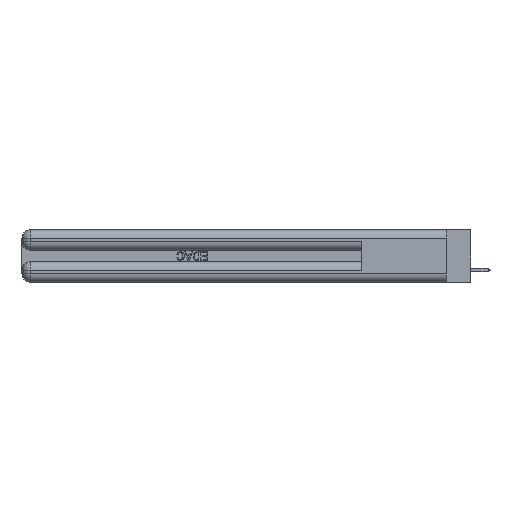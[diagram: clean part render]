
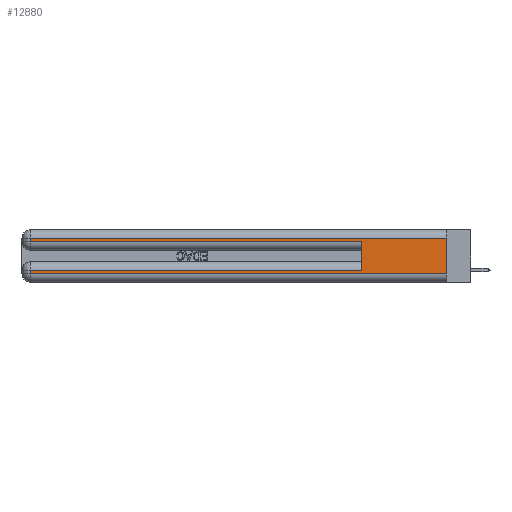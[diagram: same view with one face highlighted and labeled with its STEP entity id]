
A CAD part, left-side view. The second image highlights one B-rep face of the part: STEP entity #12880.
In plain terms, the highlighted planar face has unit normal (-1, 0, 0).
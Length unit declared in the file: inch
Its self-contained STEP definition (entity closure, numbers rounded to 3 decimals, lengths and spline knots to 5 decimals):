
#686 = EDGE_LOOP ( 'NONE', ( #40290, #36398, #44369, #18513, #11837, #49106, #40680, #31787 ) ) ;
#729 = CARTESIAN_POINT ( 'NONE',  ( 0., 0., 0.37 ) ) ;
#1629 = DIRECTION ( 'NONE',  ( 1., 0., 0. ) ) ;
#2699 = DIRECTION ( 'NONE',  ( 0., -1., 0. ) ) ;
#3109 = VECTOR ( 'NONE', #3768, 39.37008 ) ;
#3409 = VECTOR ( 'NONE', #29097, 39.37008 ) ;
#3768 = DIRECTION ( 'NONE',  ( 0., 1., 0. ) ) ;
#4962 = DIRECTION ( 'NONE',  ( 0., 0., -1. ) ) ;
#5682 = VECTOR ( 'NONE', #28118, 39.37008 ) ;
#6761 = CARTESIAN_POINT ( 'NONE',  ( 0., 2.94, 0.37 ) ) ;
#6927 = LINE ( 'NONE', #31797, #5682 ) ;
#8774 = VERTEX_POINT ( 'NONE', #41398 ) ;
#8833 = VECTOR ( 'NONE', #4962, 39.37008 ) ;
#9168 = PLANE ( 'NONE',  #35227 ) ;
#9679 = VERTEX_POINT ( 'NONE', #45547 ) ;
#10828 = VECTOR ( 'NONE', #41922, 39.37008 ) ;
#11837 = ORIENTED_EDGE ( 'NONE', *, *, #23408, .F. ) ;
#11950 = CARTESIAN_POINT ( 'NONE',  ( 0., 0., 0.31 ) ) ;
#11981 = CARTESIAN_POINT ( 'NONE',  ( 0., 2.94, 0.06 ) ) ;
#12513 = CARTESIAN_POINT ( 'NONE',  ( 0., 0., 0.085 ) ) ;
#12880 = ADVANCED_FACE ( 'NONE', ( #46481 ), #9168, .F. ) ;
#13330 = VECTOR ( 'NONE', #2699, 39.37008 ) ;
#13596 = DIRECTION ( 'NONE',  ( 0., 0., -1. ) ) ;
#17087 = VERTEX_POINT ( 'NONE', #45093 ) ;
#17309 = CARTESIAN_POINT ( 'NONE',  ( 0., 2.94, 0.085 ) ) ;
#18139 = VERTEX_POINT ( 'NONE', #26440 ) ;
#18380 = LINE ( 'NONE', #6761, #31549 ) ;
#18513 = ORIENTED_EDGE ( 'NONE', *, *, #37008, .T. ) ;
#20702 = VERTEX_POINT ( 'NONE', #29955 ) ;
#20834 = CARTESIAN_POINT ( 'NONE',  ( 0., 0., 0.37 ) ) ;
#22202 = CARTESIAN_POINT ( 'NONE',  ( 0., 2.94, 0.31 ) ) ;
#23085 = DIRECTION ( 'NONE',  ( 0., 0., -1. ) ) ;
#23408 = EDGE_CURVE ( 'NONE', #18139, #8774, #39135, .T. ) ;
#23562 = LINE ( 'NONE', #48518, #13330 ) ;
#23780 = DIRECTION ( 'NONE',  ( 0., -1., 0. ) ) ;
#23832 = LINE ( 'NONE', #12513, #3409 ) ;
#24650 = LINE ( 'NONE', #39279, #39713 ) ;
#25997 = EDGE_CURVE ( 'NONE', #27958, #32649, #18380, .T. ) ;
#26440 = CARTESIAN_POINT ( 'NONE',  ( 0., 0.6, 0.085 ) ) ;
#26708 = EDGE_CURVE ( 'NONE', #18139, #27958, #23832, .T. ) ;
#27144 = EDGE_CURVE ( 'NONE', #44528, #20702, #6927, .T. ) ;
#27958 = VERTEX_POINT ( 'NONE', #17309 ) ;
#28118 = DIRECTION ( 'NONE',  ( 0., 0., -1. ) ) ;
#29097 = DIRECTION ( 'NONE',  ( 0., 1., 0. ) ) ;
#29428 = LINE ( 'NONE', #729, #8833 ) ;
#29955 = CARTESIAN_POINT ( 'NONE',  ( 0., 2.94, 0.285 ) ) ;
#30096 = EDGE_CURVE ( 'NONE', #32649, #9679, #24650, .T. ) ;
#31350 = LINE ( 'NONE', #11950, #3109 ) ;
#31549 = VECTOR ( 'NONE', #23085, 39.37008 ) ;
#31787 = ORIENTED_EDGE ( 'NONE', *, *, #30096, .T. ) ;
#31797 = CARTESIAN_POINT ( 'NONE',  ( 0., 2.94, 0.37 ) ) ;
#32649 = VERTEX_POINT ( 'NONE', #11981 ) ;
#34162 = CARTESIAN_POINT ( 'NONE',  ( 0., 0.6, 0.145 ) ) ;
#35227 = AXIS2_PLACEMENT_3D ( 'NONE', #20834, #1629, #13596 ) ;
#36398 = ORIENTED_EDGE ( 'NONE', *, *, #42828, .T. ) ;
#37008 = EDGE_CURVE ( 'NONE', #20702, #8774, #23562, .T. ) ;
#39135 = LINE ( 'NONE', #34162, #10828 ) ;
#39279 = CARTESIAN_POINT ( 'NONE',  ( 0., 0., 0.06 ) ) ;
#39713 = VECTOR ( 'NONE', #23780, 39.37008 ) ;
#40290 = ORIENTED_EDGE ( 'NONE', *, *, #45122, .F. ) ;
#40680 = ORIENTED_EDGE ( 'NONE', *, *, #25997, .T. ) ;
#41398 = CARTESIAN_POINT ( 'NONE',  ( 0., 0.6, 0.285 ) ) ;
#41922 = DIRECTION ( 'NONE',  ( 0., 0., 1. ) ) ;
#42828 = EDGE_CURVE ( 'NONE', #17087, #44528, #31350, .T. ) ;
#44369 = ORIENTED_EDGE ( 'NONE', *, *, #27144, .T. ) ;
#44528 = VERTEX_POINT ( 'NONE', #22202 ) ;
#45093 = CARTESIAN_POINT ( 'NONE',  ( 0., 0., 0.31 ) ) ;
#45122 = EDGE_CURVE ( 'NONE', #17087, #9679, #29428, .T. ) ;
#45547 = CARTESIAN_POINT ( 'NONE',  ( 0., 0., 0.06 ) ) ;
#46481 = FACE_OUTER_BOUND ( 'NONE', #686, .T. ) ;
#48518 = CARTESIAN_POINT ( 'NONE',  ( 0., 0., 0.285 ) ) ;
#49106 = ORIENTED_EDGE ( 'NONE', *, *, #26708, .T. ) ;
